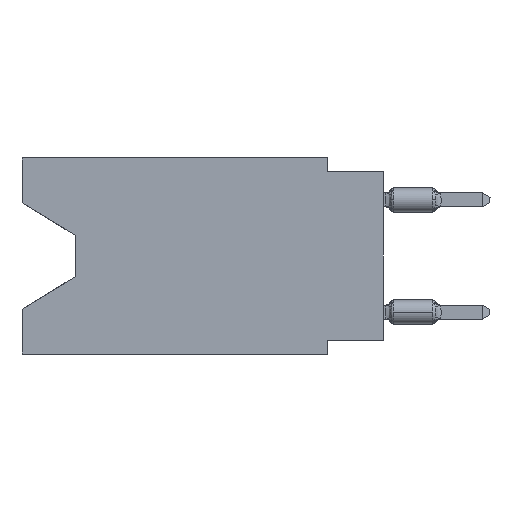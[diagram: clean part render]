
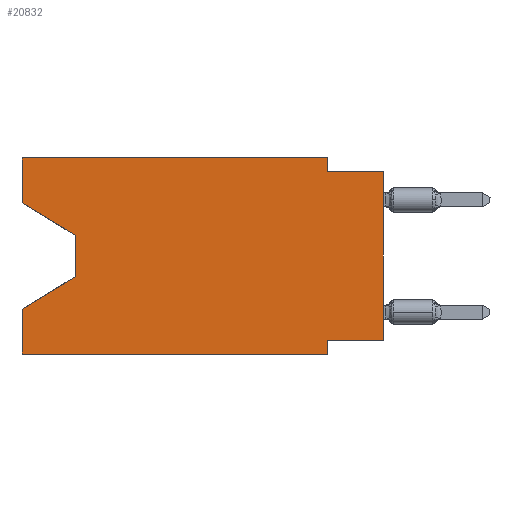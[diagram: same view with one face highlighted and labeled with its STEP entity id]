
A CAD part, left-side view. The second image highlights one B-rep face of the part: STEP entity #20832.
In plain terms, the highlighted planar face has unit normal (-1, 0, 0).
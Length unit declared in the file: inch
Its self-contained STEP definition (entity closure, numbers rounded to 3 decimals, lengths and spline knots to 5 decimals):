
#618 = FACE_OUTER_BOUND ( 'NONE', #41511, .T. ) ;
#1377 = CARTESIAN_POINT ( 'NONE',  ( 0., 0.645, 0. ) ) ;
#1447 = CARTESIAN_POINT ( 'NONE',  ( 0., 0.645, -0.35 ) ) ;
#1570 = CARTESIAN_POINT ( 'NONE',  ( 0., 0., -0.325 ) ) ;
#1896 = CARTESIAN_POINT ( 'NONE',  ( 0., 0.1, -0.025 ) ) ;
#1927 = DIRECTION ( 'NONE',  ( 0., -1., 0. ) ) ;
#2083 = CARTESIAN_POINT ( 'NONE',  ( 0., 0.1, -0.325 ) ) ;
#2717 = CARTESIAN_POINT ( 'NONE',  ( 0., 0.645, -0.26975 ) ) ;
#3611 = VECTOR ( 'NONE', #40483, 39.37008 ) ;
#3700 = CARTESIAN_POINT ( 'NONE',  ( 0., 0.645, 0. ) ) ;
#3707 = ORIENTED_EDGE ( 'NONE', *, *, #29903, .F. ) ;
#3910 = VERTEX_POINT ( 'NONE', #46453 ) ;
#3953 = LINE ( 'NONE', #3700, #15477 ) ;
#5005 = LINE ( 'NONE', #28997, #3611 ) ;
#5102 = CARTESIAN_POINT ( 'NONE',  ( 0., 0.55, -0.212 ) ) ;
#5575 = ORIENTED_EDGE ( 'NONE', *, *, #40534, .F. ) ;
#5635 = EDGE_CURVE ( 'NONE', #41653, #26834, #19051, .T. ) ;
#6497 = EDGE_CURVE ( 'NONE', #21473, #25921, #44659, .T. ) ;
#6798 = ORIENTED_EDGE ( 'NONE', *, *, #27615, .F. ) ;
#7573 = CARTESIAN_POINT ( 'NONE',  ( 0., 0.55, -0.212 ) ) ;
#8108 = VECTOR ( 'NONE', #10988, 39.37008 ) ;
#8962 = DIRECTION ( 'NONE',  ( 0., 0., -1. ) ) ;
#9596 = VERTEX_POINT ( 'NONE', #2083 ) ;
#10520 = CARTESIAN_POINT ( 'NONE',  ( 0., 0., -0.025 ) ) ;
#10645 = LINE ( 'NONE', #30471, #39534 ) ;
#10683 = VECTOR ( 'NONE', #41787, 39.37008 ) ;
#10988 = DIRECTION ( 'NONE',  ( 0., 0.855, -0.519 ) ) ;
#12114 = CARTESIAN_POINT ( 'NONE',  ( 0., 0.55, -0.138 ) ) ;
#13025 = EDGE_CURVE ( 'NONE', #21473, #9596, #5005, .T. ) ;
#13251 = VECTOR ( 'NONE', #23051, 39.37008 ) ;
#13808 = CARTESIAN_POINT ( 'NONE',  ( 0., 0.645, 0. ) ) ;
#13951 = DIRECTION ( 'NONE',  ( 0., 0., -1. ) ) ;
#14319 = EDGE_CURVE ( 'NONE', #3910, #15162, #10645, .T. ) ;
#14996 = ORIENTED_EDGE ( 'NONE', *, *, #33478, .T. ) ;
#15162 = VERTEX_POINT ( 'NONE', #12114 ) ;
#15477 = VECTOR ( 'NONE', #16463, 39.37008 ) ;
#15918 = EDGE_CURVE ( 'NONE', #3910, #34191, #23163, .T. ) ;
#16004 = ORIENTED_EDGE ( 'NONE', *, *, #48595, .F. ) ;
#16463 = DIRECTION ( 'NONE',  ( 0., 0., 1. ) ) ;
#16910 = DIRECTION ( 'NONE',  ( 0., 0., -1. ) ) ;
#18032 = ORIENTED_EDGE ( 'NONE', *, *, #6497, .T. ) ;
#18939 = VECTOR ( 'NONE', #13951, 39.37008 ) ;
#19051 = LINE ( 'NONE', #7573, #8108 ) ;
#20832 = ADVANCED_FACE ( 'NONE', ( #618 ), #36618, .F. ) ;
#20959 = VECTOR ( 'NONE', #16910, 39.37008 ) ;
#21349 = LINE ( 'NONE', #40921, #20959 ) ;
#21473 = VERTEX_POINT ( 'NONE', #1570 ) ;
#22216 = CARTESIAN_POINT ( 'NONE',  ( 0., 0.55, -0.138 ) ) ;
#22716 = ORIENTED_EDGE ( 'NONE', *, *, #13025, .F. ) ;
#23051 = DIRECTION ( 'NONE',  ( 0., -1., 0. ) ) ;
#23163 = LINE ( 'NONE', #47405, #37938 ) ;
#23311 = LINE ( 'NONE', #47287, #13251 ) ;
#24623 = DIRECTION ( 'NONE',  ( 1., 0., 0. ) ) ;
#25921 = VERTEX_POINT ( 'NONE', #36945 ) ;
#26133 = DIRECTION ( 'NONE',  ( 0., 0., -1. ) ) ;
#26215 = LINE ( 'NONE', #37452, #18939 ) ;
#26563 = DIRECTION ( 'NONE',  ( 0., -0.855, -0.519 ) ) ;
#26834 = VERTEX_POINT ( 'NONE', #2717 ) ;
#27085 = DIRECTION ( 'NONE',  ( 0., 0., 1. ) ) ;
#27615 = EDGE_CURVE ( 'NONE', #27646, #30293, #21349, .T. ) ;
#27646 = VERTEX_POINT ( 'NONE', #28916 ) ;
#28043 = VERTEX_POINT ( 'NONE', #1447 ) ;
#28264 = AXIS2_PLACEMENT_3D ( 'NONE', #1377, #24623, #8962 ) ;
#28916 = CARTESIAN_POINT ( 'NONE',  ( 0., 0.1, 0. ) ) ;
#28997 = CARTESIAN_POINT ( 'NONE',  ( 0., 0., -0.325 ) ) ;
#29903 = EDGE_CURVE ( 'NONE', #9596, #50969, #26215, .T. ) ;
#30293 = VERTEX_POINT ( 'NONE', #1896 ) ;
#30471 = CARTESIAN_POINT ( 'NONE',  ( 0., 0.645, -0.08025 ) ) ;
#33478 = EDGE_CURVE ( 'NONE', #28043, #50969, #23311, .T. ) ;
#33842 = CARTESIAN_POINT ( 'NONE',  ( 0., 0.1, -0.35 ) ) ;
#34001 = LINE ( 'NONE', #10520, #48061 ) ;
#34191 = VERTEX_POINT ( 'NONE', #13808 ) ;
#35635 = EDGE_CURVE ( 'NONE', #15162, #41653, #45432, .T. ) ;
#36618 = PLANE ( 'NONE',  #28264 ) ;
#36945 = CARTESIAN_POINT ( 'NONE',  ( 0., 0., -0.025 ) ) ;
#37357 = DIRECTION ( 'NONE',  ( 0., 0., 1. ) ) ;
#37452 = CARTESIAN_POINT ( 'NONE',  ( 0., 0.1, -0.35 ) ) ;
#37560 = VECTOR ( 'NONE', #26133, 39.37008 ) ;
#37938 = VECTOR ( 'NONE', #27085, 39.37008 ) ;
#38040 = ORIENTED_EDGE ( 'NONE', *, *, #15918, .F. ) ;
#39534 = VECTOR ( 'NONE', #26563, 39.37008 ) ;
#40483 = DIRECTION ( 'NONE',  ( 0., 1., 0. ) ) ;
#40534 = EDGE_CURVE ( 'NONE', #30293, #25921, #34001, .T. ) ;
#40921 = CARTESIAN_POINT ( 'NONE',  ( 0., 0.1, 0. ) ) ;
#41477 = VECTOR ( 'NONE', #37357, 39.37008 ) ;
#41511 = EDGE_LOOP ( 'NONE', ( #48845, #50808, #41907, #16004, #14996, #3707, #22716, #18032, #5575, #6798, #42801, #38040 ) ) ;
#41653 = VERTEX_POINT ( 'NONE', #5102 ) ;
#41787 = DIRECTION ( 'NONE',  ( 0., -1., 0. ) ) ;
#41907 = ORIENTED_EDGE ( 'NONE', *, *, #5635, .T. ) ;
#42251 = EDGE_CURVE ( 'NONE', #34191, #27646, #45944, .T. ) ;
#42801 = ORIENTED_EDGE ( 'NONE', *, *, #42251, .F. ) ;
#44659 = LINE ( 'NONE', #44920, #41477 ) ;
#44920 = CARTESIAN_POINT ( 'NONE',  ( 0., 0., 0. ) ) ;
#45432 = LINE ( 'NONE', #22216, #37560 ) ;
#45944 = LINE ( 'NONE', #50356, #10683 ) ;
#46453 = CARTESIAN_POINT ( 'NONE',  ( 0., 0.645, -0.08025 ) ) ;
#47287 = CARTESIAN_POINT ( 'NONE',  ( 0., 0.645, -0.35 ) ) ;
#47405 = CARTESIAN_POINT ( 'NONE',  ( 0., 0.645, 0. ) ) ;
#48061 = VECTOR ( 'NONE', #1927, 39.37008 ) ;
#48595 = EDGE_CURVE ( 'NONE', #28043, #26834, #3953, .T. ) ;
#48845 = ORIENTED_EDGE ( 'NONE', *, *, #14319, .T. ) ;
#50356 = CARTESIAN_POINT ( 'NONE',  ( 0., 0.645, 0. ) ) ;
#50808 = ORIENTED_EDGE ( 'NONE', *, *, #35635, .T. ) ;
#50969 = VERTEX_POINT ( 'NONE', #33842 ) ;
